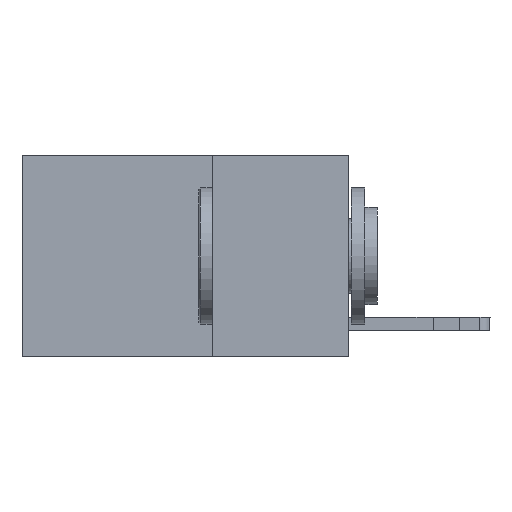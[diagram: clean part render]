
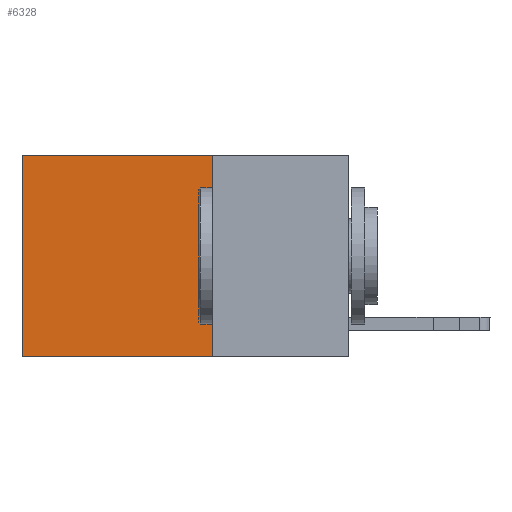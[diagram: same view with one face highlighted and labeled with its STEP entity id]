
A CAD part, left-side view. The second image highlights one B-rep face of the part: STEP entity #6328.
In plain terms, the highlighted planar face has unit normal (-1, 0, 0).
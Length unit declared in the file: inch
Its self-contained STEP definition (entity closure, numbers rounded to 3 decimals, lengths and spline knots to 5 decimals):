
#159 = VERTEX_POINT ( 'NONE', #3439 ) ;
#435 = EDGE_CURVE ( 'NONE', #159, #2015, #5569, .T. ) ;
#600 = ORIENTED_EDGE ( 'NONE', *, *, #13570, .T. ) ;
#786 = LINE ( 'NONE', #15954, #7393 ) ;
#1259 = CARTESIAN_POINT ( 'NONE',  ( 0.2625, 0.6, -0.37 ) ) ;
#1319 = ORIENTED_EDGE ( 'NONE', *, *, #5924, .T. ) ;
#1893 = DIRECTION ( 'NONE',  ( 1., 0., 0. ) ) ;
#2015 = VERTEX_POINT ( 'NONE', #1259 ) ;
#2987 = CARTESIAN_POINT ( 'NONE',  ( 0.2625, 0.25, -0.37 ) ) ;
#3439 = CARTESIAN_POINT ( 'NONE',  ( 0.2625, 0.25, -0.37 ) ) ;
#3445 = AXIS2_PLACEMENT_3D ( 'NONE', #15498, #1893, #14494 ) ;
#3944 = VECTOR ( 'NONE', #4480, 39.37008 ) ;
#4198 = LINE ( 'NONE', #10413, #15234 ) ;
#4480 = DIRECTION ( 'NONE',  ( 0., 0., -1. ) ) ;
#5478 = EDGE_CURVE ( 'NONE', #12792, #159, #786, .T. ) ;
#5569 = LINE ( 'NONE', #2987, #10513 ) ;
#5924 = EDGE_CURVE ( 'NONE', #12531, #2015, #9284, .T. ) ;
#6328 = ADVANCED_FACE ( 'NONE', ( #11912 ), #13241, .F. ) ;
#7393 = VECTOR ( 'NONE', #9634, 39.37008 ) ;
#8223 = CARTESIAN_POINT ( 'NONE',  ( 0.2625, 0.6, 0. ) ) ;
#8829 = ORIENTED_EDGE ( 'NONE', *, *, #435, .F. ) ;
#9284 = LINE ( 'NONE', #8223, #3944 ) ;
#9304 = EDGE_LOOP ( 'NONE', ( #1319, #8829, #10537, #600 ) ) ;
#9634 = DIRECTION ( 'NONE',  ( 0., 0., -1. ) ) ;
#10413 = CARTESIAN_POINT ( 'NONE',  ( 0.2625, 0.25, 0. ) ) ;
#10513 = VECTOR ( 'NONE', #15598, 39.37008 ) ;
#10537 = ORIENTED_EDGE ( 'NONE', *, *, #5478, .F. ) ;
#11624 = CARTESIAN_POINT ( 'NONE',  ( 0.2625, 0.25, 0. ) ) ;
#11812 = DIRECTION ( 'NONE',  ( 0., 1., 0. ) ) ;
#11912 = FACE_OUTER_BOUND ( 'NONE', #9304, .T. ) ;
#12531 = VERTEX_POINT ( 'NONE', #14986 ) ;
#12792 = VERTEX_POINT ( 'NONE', #11624 ) ;
#13241 = PLANE ( 'NONE',  #3445 ) ;
#13570 = EDGE_CURVE ( 'NONE', #12792, #12531, #4198, .T. ) ;
#14494 = DIRECTION ( 'NONE',  ( 0., 0., -1. ) ) ;
#14986 = CARTESIAN_POINT ( 'NONE',  ( 0.2625, 0.6, 0. ) ) ;
#15234 = VECTOR ( 'NONE', #11812, 39.37008 ) ;
#15498 = CARTESIAN_POINT ( 'NONE',  ( 0.2625, 0.25, 0. ) ) ;
#15598 = DIRECTION ( 'NONE',  ( 0., 1., 0. ) ) ;
#15954 = CARTESIAN_POINT ( 'NONE',  ( 0.2625, 0.25, 0. ) ) ;
